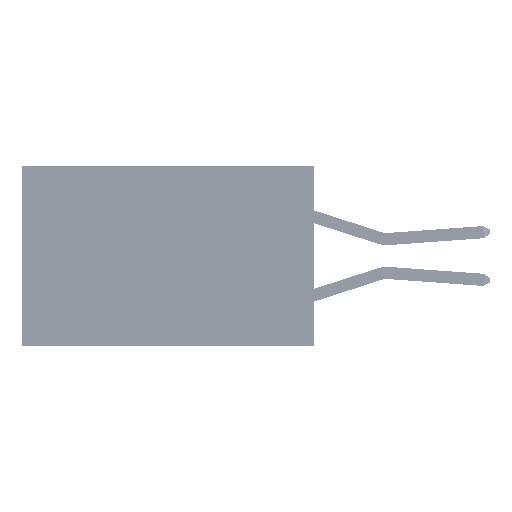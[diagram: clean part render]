
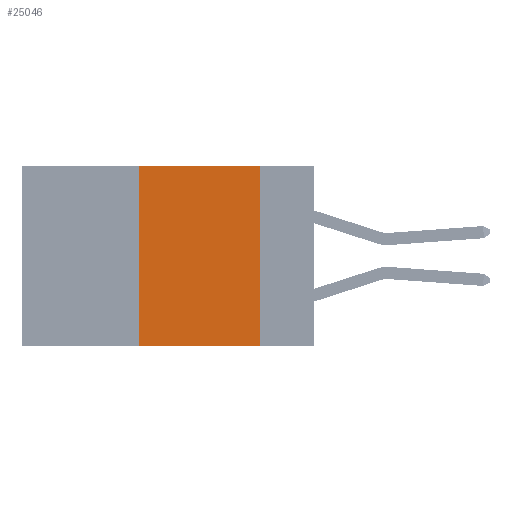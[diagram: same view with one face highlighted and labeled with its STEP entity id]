
A CAD part, left-side view. The second image highlights one B-rep face of the part: STEP entity #25046.
In plain terms, the highlighted planar face has unit normal (-1, 0, 0).
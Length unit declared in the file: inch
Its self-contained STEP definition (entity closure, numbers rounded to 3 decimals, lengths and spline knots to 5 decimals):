
#375 = ORIENTED_EDGE ( 'NONE', *, *, #37407, .F. ) ;
#1862 = CARTESIAN_POINT ( 'NONE',  ( 0., 0.36, 0. ) ) ;
#6535 = EDGE_CURVE ( 'NONE', #37305, #13934, #50920, .T. ) ;
#7011 = VERTEX_POINT ( 'NONE', #1862 ) ;
#7941 = LINE ( 'NONE', #32762, #19885 ) ;
#12268 = DIRECTION ( 'NONE',  ( 1., 0., 0. ) ) ;
#13342 = CARTESIAN_POINT ( 'NONE',  ( 0., 0.11, 0. ) ) ;
#13934 = VERTEX_POINT ( 'NONE', #24342 ) ;
#14047 = CARTESIAN_POINT ( 'NONE',  ( 0., 0.6, -0.37 ) ) ;
#15341 = EDGE_CURVE ( 'NONE', #7011, #40079, #7941, .T. ) ;
#17545 = CARTESIAN_POINT ( 'NONE',  ( 0., 0.36, 0. ) ) ;
#19560 = VECTOR ( 'NONE', #30063, 39.37008 ) ;
#19856 = CARTESIAN_POINT ( 'NONE',  ( 0., 0.6, 0. ) ) ;
#19861 = EDGE_LOOP ( 'NONE', ( #375, #52857, #30855, #26554 ) ) ;
#19885 = VECTOR ( 'NONE', #27398, 39.37008 ) ;
#21074 = DIRECTION ( 'NONE',  ( 0., 0., 1. ) ) ;
#23703 = VECTOR ( 'NONE', #30486, 39.37008 ) ;
#24342 = CARTESIAN_POINT ( 'NONE',  ( 0., 0.11, -0.37 ) ) ;
#25046 = ADVANCED_FACE ( 'NONE', ( #52391 ), #45135, .F. ) ;
#26554 = ORIENTED_EDGE ( 'NONE', *, *, #6535, .T. ) ;
#27398 = DIRECTION ( 'NONE',  ( 0., -1., 0. ) ) ;
#29217 = VECTOR ( 'NONE', #21074, 39.37008 ) ;
#30063 = DIRECTION ( 'NONE',  ( 0., 0., -1. ) ) ;
#30486 = DIRECTION ( 'NONE',  ( 0., -1., 0. ) ) ;
#30855 = ORIENTED_EDGE ( 'NONE', *, *, #52024, .F. ) ;
#32762 = CARTESIAN_POINT ( 'NONE',  ( 0., 0.6, 0. ) ) ;
#36244 = DIRECTION ( 'NONE',  ( 0., 0., -1. ) ) ;
#37305 = VERTEX_POINT ( 'NONE', #40832 ) ;
#37407 = EDGE_CURVE ( 'NONE', #40079, #13934, #51017, .T. ) ;
#40079 = VERTEX_POINT ( 'NONE', #52690 ) ;
#40832 = CARTESIAN_POINT ( 'NONE',  ( 0., 0.36, -0.37 ) ) ;
#43309 = AXIS2_PLACEMENT_3D ( 'NONE', #19856, #12268, #36244 ) ;
#45135 = PLANE ( 'NONE',  #43309 ) ;
#46072 = LINE ( 'NONE', #17545, #29217 ) ;
#50920 = LINE ( 'NONE', #14047, #23703 ) ;
#51017 = LINE ( 'NONE', #13342, #19560 ) ;
#52024 = EDGE_CURVE ( 'NONE', #37305, #7011, #46072, .T. ) ;
#52391 = FACE_OUTER_BOUND ( 'NONE', #19861, .T. ) ;
#52690 = CARTESIAN_POINT ( 'NONE',  ( 0., 0.11, 0. ) ) ;
#52857 = ORIENTED_EDGE ( 'NONE', *, *, #15341, .F. ) ;
